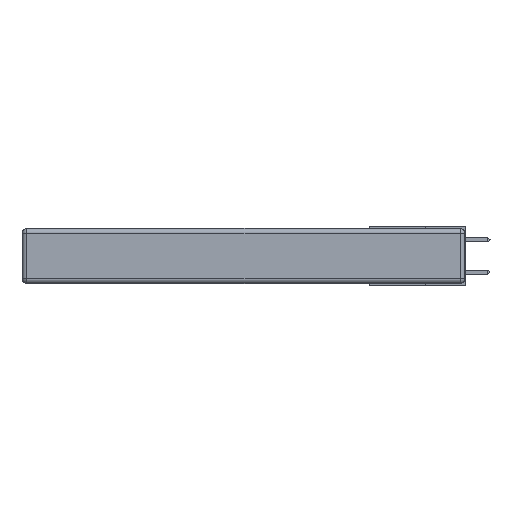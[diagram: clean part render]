
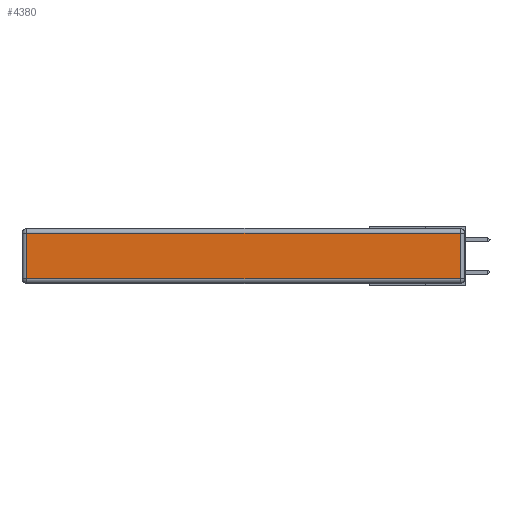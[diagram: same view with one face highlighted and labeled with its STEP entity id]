
A CAD part, left-side view. The second image highlights one B-rep face of the part: STEP entity #4380.
In plain terms, the highlighted planar face has unit normal (-1, 0, 0).
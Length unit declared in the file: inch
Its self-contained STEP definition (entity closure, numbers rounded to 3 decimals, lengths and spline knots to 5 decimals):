
#1371 = VERTEX_POINT ( 'NONE', #5805 ) ;
#1544 = CARTESIAN_POINT ( 'NONE',  ( 0., 2.72, -0.313 ) ) ;
#3549 = EDGE_CURVE ( 'NONE', #17901, #4107, #18882, .T. ) ;
#3744 = DIRECTION ( 'NONE',  ( 0., 1., 0. ) ) ;
#3854 = EDGE_CURVE ( 'NONE', #16955, #1371, #22243, .T. ) ;
#4107 = VERTEX_POINT ( 'NONE', #4520 ) ;
#4380 = ADVANCED_FACE ( 'NONE', ( #8274 ), #10338, .T. ) ;
#4390 = DIRECTION ( 'NONE',  ( 0., 0., -1. ) ) ;
#4487 = VECTOR ( 'NONE', #4390, 39.37008 ) ;
#4520 = CARTESIAN_POINT ( 'NONE',  ( 0., 0.03, -0.313 ) ) ;
#4951 = VECTOR ( 'NONE', #12573, 39.37008 ) ;
#5805 = CARTESIAN_POINT ( 'NONE',  ( 0., 2.72, -0.03 ) ) ;
#5945 = EDGE_LOOP ( 'NONE', ( #12124, #13850, #17447, #9822 ) ) ;
#6668 = DIRECTION ( 'NONE',  ( -1., 0., 0. ) ) ;
#6832 = CARTESIAN_POINT ( 'NONE',  ( 0., 0.03, -0.343 ) ) ;
#8274 = FACE_OUTER_BOUND ( 'NONE', #5945, .T. ) ;
#8686 = CARTESIAN_POINT ( 'NONE',  ( 0., 0.03, -0.03 ) ) ;
#8995 = DIRECTION ( 'NONE',  ( 0., 0., 1. ) ) ;
#9822 = ORIENTED_EDGE ( 'NONE', *, *, #14847, .T. ) ;
#10338 = PLANE ( 'NONE',  #12963 ) ;
#10363 = LINE ( 'NONE', #11346, #4487 ) ;
#11346 = CARTESIAN_POINT ( 'NONE',  ( 0., 2.72, -0.343 ) ) ;
#11907 = EDGE_CURVE ( 'NONE', #4107, #16955, #19377, .T. ) ;
#12124 = ORIENTED_EDGE ( 'NONE', *, *, #3549, .T. ) ;
#12455 = VECTOR ( 'NONE', #3744, 39.37008 ) ;
#12573 = DIRECTION ( 'NONE',  ( 0., -1., 0. ) ) ;
#12963 = AXIS2_PLACEMENT_3D ( 'NONE', #17458, #6668, #8995 ) ;
#13243 = VECTOR ( 'NONE', #22744, 39.37008 ) ;
#13850 = ORIENTED_EDGE ( 'NONE', *, *, #11907, .T. ) ;
#14847 = EDGE_CURVE ( 'NONE', #1371, #17901, #10363, .T. ) ;
#16955 = VERTEX_POINT ( 'NONE', #8686 ) ;
#17447 = ORIENTED_EDGE ( 'NONE', *, *, #3854, .T. ) ;
#17458 = CARTESIAN_POINT ( 'NONE',  ( 0., 0., -0.343 ) ) ;
#17901 = VERTEX_POINT ( 'NONE', #1544 ) ;
#18882 = LINE ( 'NONE', #21384, #4951 ) ;
#19377 = LINE ( 'NONE', #6832, #13243 ) ;
#21369 = CARTESIAN_POINT ( 'NONE',  ( 0., 2.75, -0.03 ) ) ;
#21384 = CARTESIAN_POINT ( 'NONE',  ( 0., 0., -0.313 ) ) ;
#22243 = LINE ( 'NONE', #21369, #12455 ) ;
#22744 = DIRECTION ( 'NONE',  ( 0., 0., 1. ) ) ;
